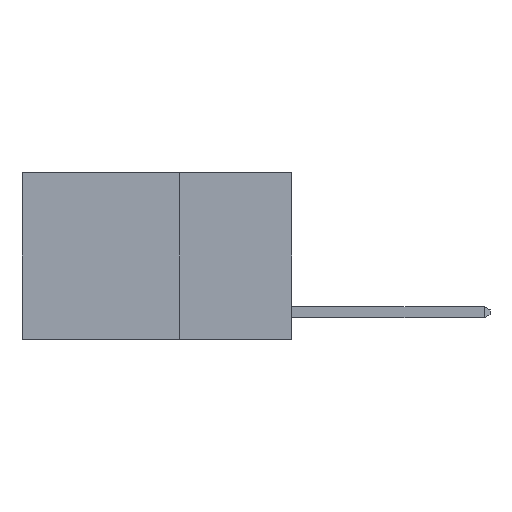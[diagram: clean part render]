
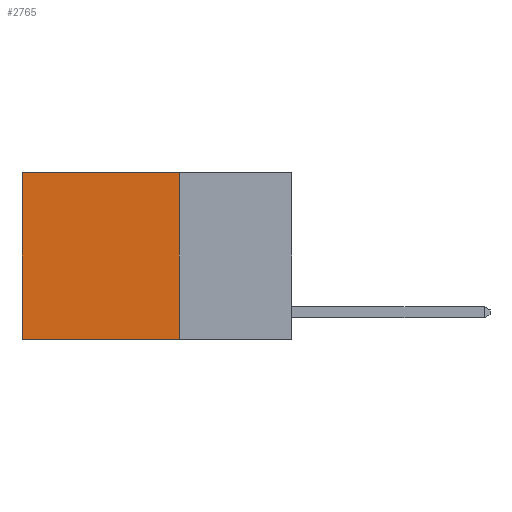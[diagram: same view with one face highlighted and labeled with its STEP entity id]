
A CAD part, left-side view. The second image highlights one B-rep face of the part: STEP entity #2765.
In plain terms, the highlighted planar face has unit normal (-1, 0, 0).
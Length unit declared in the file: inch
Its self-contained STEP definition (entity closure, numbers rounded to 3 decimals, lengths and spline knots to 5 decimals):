
#679 = CARTESIAN_POINT ( 'NONE',  ( 0.2625, 0.6, -0.37 ) ) ;
#817 = ORIENTED_EDGE ( 'NONE', *, *, #868, .T. ) ;
#868 = EDGE_CURVE ( 'NONE', #7213, #10017, #3125, .T. ) ;
#1330 = LINE ( 'NONE', #8165, #9928 ) ;
#1346 = VERTEX_POINT ( 'NONE', #679 ) ;
#1581 = DIRECTION ( 'NONE',  ( 0., 0., -1. ) ) ;
#1822 = CARTESIAN_POINT ( 'NONE',  ( 0.2625, 0.6, 0. ) ) ;
#2031 = EDGE_CURVE ( 'NONE', #7213, #10486, #4643, .T. ) ;
#2623 = EDGE_CURVE ( 'NONE', #10486, #1346, #1330, .T. ) ;
#2665 = CARTESIAN_POINT ( 'NONE',  ( 0.2625, 0.25, 0. ) ) ;
#2765 = ADVANCED_FACE ( 'NONE', ( #8733 ), #9129, .F. ) ;
#3125 = LINE ( 'NONE', #3490, #9496 ) ;
#3381 = DIRECTION ( 'NONE',  ( 0., 1., 0. ) ) ;
#3490 = CARTESIAN_POINT ( 'NONE',  ( 0.2625, 0.25, 0. ) ) ;
#4164 = ORIENTED_EDGE ( 'NONE', *, *, #2031, .F. ) ;
#4368 = CARTESIAN_POINT ( 'NONE',  ( 0.2625, 0.25, 0. ) ) ;
#4643 = LINE ( 'NONE', #10437, #8625 ) ;
#5034 = ORIENTED_EDGE ( 'NONE', *, *, #2623, .F. ) ;
#5162 = EDGE_CURVE ( 'NONE', #10017, #1346, #6012, .T. ) ;
#5217 = DIRECTION ( 'NONE',  ( 0., 0., -1. ) ) ;
#6012 = LINE ( 'NONE', #1822, #8065 ) ;
#6402 = CARTESIAN_POINT ( 'NONE',  ( 0.2625, 0.25, -0.37 ) ) ;
#6752 = AXIS2_PLACEMENT_3D ( 'NONE', #4368, #9902, #5217 ) ;
#6765 = DIRECTION ( 'NONE',  ( 0., 0., -1. ) ) ;
#7037 = ORIENTED_EDGE ( 'NONE', *, *, #5162, .T. ) ;
#7213 = VERTEX_POINT ( 'NONE', #2665 ) ;
#8026 = CARTESIAN_POINT ( 'NONE',  ( 0.2625, 0.6, 0. ) ) ;
#8065 = VECTOR ( 'NONE', #6765, 39.37008 ) ;
#8165 = CARTESIAN_POINT ( 'NONE',  ( 0.2625, 0.25, -0.37 ) ) ;
#8625 = VECTOR ( 'NONE', #1581, 39.37008 ) ;
#8733 = FACE_OUTER_BOUND ( 'NONE', #9676, .T. ) ;
#9129 = PLANE ( 'NONE',  #6752 ) ;
#9496 = VECTOR ( 'NONE', #9834, 39.37008 ) ;
#9676 = EDGE_LOOP ( 'NONE', ( #7037, #5034, #4164, #817 ) ) ;
#9834 = DIRECTION ( 'NONE',  ( 0., 1., 0. ) ) ;
#9902 = DIRECTION ( 'NONE',  ( 1., 0., 0. ) ) ;
#9928 = VECTOR ( 'NONE', #3381, 39.37008 ) ;
#10017 = VERTEX_POINT ( 'NONE', #8026 ) ;
#10437 = CARTESIAN_POINT ( 'NONE',  ( 0.2625, 0.25, 0. ) ) ;
#10486 = VERTEX_POINT ( 'NONE', #6402 ) ;
